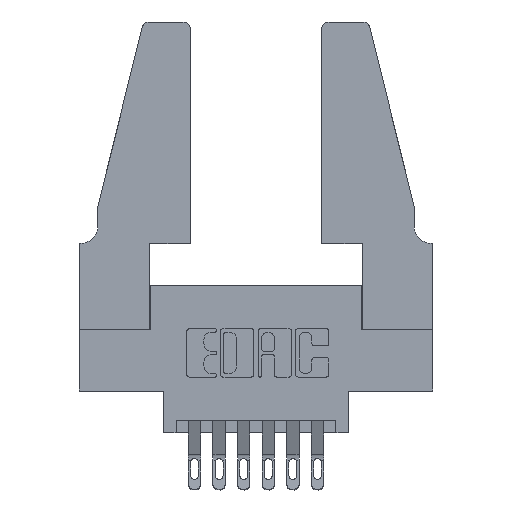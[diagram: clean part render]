
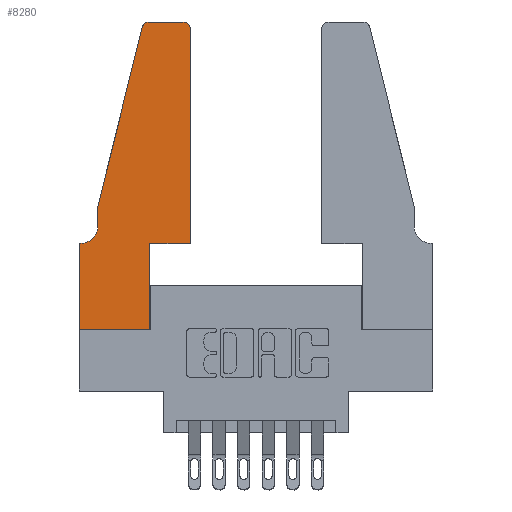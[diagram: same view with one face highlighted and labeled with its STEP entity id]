
A CAD part, top view. The second image highlights one B-rep face of the part: STEP entity #8280.
In plain terms, the highlighted planar face has unit normal (0, 0, 1).
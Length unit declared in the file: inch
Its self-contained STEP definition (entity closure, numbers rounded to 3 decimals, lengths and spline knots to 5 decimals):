
#28 = VECTOR ( 'NONE', #270, 39.37008 ) ;
#76 = CIRCLE ( 'NONE', #6480, 0.03 ) ;
#229 = VERTEX_POINT ( 'NONE', #832 ) ;
#270 = DIRECTION ( 'NONE',  ( -0.239, -0.971, 0. ) ) ;
#282 = CARTESIAN_POINT ( 'NONE',  ( 0.0755, 0.5, 0.37 ) ) ;
#546 = LINE ( 'NONE', #2234, #886 ) ;
#561 = CARTESIAN_POINT ( 'NONE',  ( 0.2865, 0.35, 0.37 ) ) ;
#663 = VERTEX_POINT ( 'NONE', #5382 ) ;
#832 = CARTESIAN_POINT ( 'NONE',  ( 0.0755, 0.5, 0.37 ) ) ;
#846 = EDGE_CURVE ( 'NONE', #4958, #2018, #1470, .T. ) ;
#886 = VECTOR ( 'NONE', #2014, 39.37008 ) ;
#1030 = CARTESIAN_POINT ( 'NONE',  ( 0., 0.35, 0.37 ) ) ;
#1070 = ORIENTED_EDGE ( 'NONE', *, *, #9901, .T. ) ;
#1349 = VERTEX_POINT ( 'NONE', #561 ) ;
#1470 = LINE ( 'NONE', #11175, #6587 ) ;
#1544 = CARTESIAN_POINT ( 'NONE',  ( 0., 0.35, 0.37 ) ) ;
#1828 = ORIENTED_EDGE ( 'NONE', *, *, #3457, .T. ) ;
#1980 = DIRECTION ( 'NONE',  ( 0., 0., 1. ) ) ;
#2014 = DIRECTION ( 'NONE',  ( 1., 0., 0. ) ) ;
#2018 = VERTEX_POINT ( 'NONE', #7137 ) ;
#2154 = CARTESIAN_POINT ( 'NONE',  ( 0.0755, 0.42, 0.37 ) ) ;
#2234 = CARTESIAN_POINT ( 'NONE',  ( 0.4505, 0.35, 0.37 ) ) ;
#2281 = CARTESIAN_POINT ( 'NONE',  ( 0.4205, 1.22, 0.37 ) ) ;
#2283 = EDGE_LOOP ( 'NONE', ( #7116, #5457, #11594, #6829, #2552, #1828, #3752, #1070, #11654, #7607, #7612, #5380 ) ) ;
#2552 = ORIENTED_EDGE ( 'NONE', *, *, #4935, .T. ) ;
#2632 = CIRCLE ( 'NONE', #11455, 0.03 ) ;
#2892 = DIRECTION ( 'NONE',  ( -1., 0., 0. ) ) ;
#2947 = VERTEX_POINT ( 'NONE', #3494 ) ;
#2970 = CARTESIAN_POINT ( 'NONE',  ( 0.0055, 0.42, 0.37 ) ) ;
#3032 = DIRECTION ( 'NONE',  ( 0., -1., 0. ) ) ;
#3078 = DIRECTION ( 'NONE',  ( 0., 0., -1. ) ) ;
#3112 = CARTESIAN_POINT ( 'NONE',  ( 0.25487, 1.22718, 0.37 ) ) ;
#3214 = DIRECTION ( 'NONE',  ( 1., 0., 0. ) ) ;
#3267 = EDGE_CURVE ( 'NONE', #663, #5713, #5959, .T. ) ;
#3369 = LINE ( 'NONE', #282, #28 ) ;
#3457 = EDGE_CURVE ( 'NONE', #9056, #4958, #6723, .T. ) ;
#3494 = CARTESIAN_POINT ( 'NONE',  ( 0.4505, 0.35, 0.37 ) ) ;
#3605 = AXIS2_PLACEMENT_3D ( 'NONE', #1030, #4929, #11365 ) ;
#3752 = ORIENTED_EDGE ( 'NONE', *, *, #846, .T. ) ;
#4354 = FACE_OUTER_BOUND ( 'NONE', #2283, .T. ) ;
#4867 = EDGE_CURVE ( 'NONE', #1349, #2947, #546, .T. ) ;
#4929 = DIRECTION ( 'NONE',  ( 0., 0., 1. ) ) ;
#4935 = EDGE_CURVE ( 'NONE', #7271, #9056, #5158, .T. ) ;
#4958 = VERTEX_POINT ( 'NONE', #1544 ) ;
#5158 = CIRCLE ( 'NONE', #7493, 0.07 ) ;
#5163 = EDGE_CURVE ( 'NONE', #5981, #229, #3369, .T. ) ;
#5170 = DIRECTION ( 'NONE',  ( 0., 1., 0. ) ) ;
#5186 = LINE ( 'NONE', #6149, #9880 ) ;
#5211 = VECTOR ( 'NONE', #7538, 39.37008 ) ;
#5380 = ORIENTED_EDGE ( 'NONE', *, *, #5427, .T. ) ;
#5382 = CARTESIAN_POINT ( 'NONE',  ( 0.4205, 1.25, 0.37 ) ) ;
#5427 = EDGE_CURVE ( 'NONE', #6000, #663, #2632, .T. ) ;
#5457 = ORIENTED_EDGE ( 'NONE', *, *, #10553, .T. ) ;
#5499 = VECTOR ( 'NONE', #5170, 39.37008 ) ;
#5713 = VERTEX_POINT ( 'NONE', #11856 ) ;
#5959 = LINE ( 'NONE', #8402, #10574 ) ;
#5981 = VERTEX_POINT ( 'NONE', #3112 ) ;
#6000 = VERTEX_POINT ( 'NONE', #6984 ) ;
#6149 = CARTESIAN_POINT ( 'NONE',  ( 0.0755, 0.5, 0.37 ) ) ;
#6259 = CARTESIAN_POINT ( 'NONE',  ( 0.4505, 0.35, 0.37 ) ) ;
#6480 = AXIS2_PLACEMENT_3D ( 'NONE', #7685, #1980, #8608 ) ;
#6587 = VECTOR ( 'NONE', #3032, 39.37008 ) ;
#6723 = LINE ( 'NONE', #10521, #8886 ) ;
#6829 = ORIENTED_EDGE ( 'NONE', *, *, #10794, .T. ) ;
#6984 = CARTESIAN_POINT ( 'NONE',  ( 0.4505, 1.22, 0.37 ) ) ;
#7116 = ORIENTED_EDGE ( 'NONE', *, *, #3267, .T. ) ;
#7130 = DIRECTION ( 'NONE',  ( 0., -1., 0. ) ) ;
#7137 = CARTESIAN_POINT ( 'NONE',  ( 0., 0., 0.37 ) ) ;
#7271 = VERTEX_POINT ( 'NONE', #2154 ) ;
#7493 = AXIS2_PLACEMENT_3D ( 'NONE', #2970, #3078, #2892 ) ;
#7524 = VERTEX_POINT ( 'NONE', #11751 ) ;
#7538 = DIRECTION ( 'NONE',  ( 1., 0., 0. ) ) ;
#7607 = ORIENTED_EDGE ( 'NONE', *, *, #4867, .T. ) ;
#7612 = ORIENTED_EDGE ( 'NONE', *, *, #8497, .T. ) ;
#7685 = CARTESIAN_POINT ( 'NONE',  ( 0.284, 1.22, 0.37 ) ) ;
#8007 = CARTESIAN_POINT ( 'NONE',  ( 0.2865, 0.35, 0.37 ) ) ;
#8021 = LINE ( 'NONE', #8007, #5499 ) ;
#8045 = LINE ( 'NONE', #9336, #5211 ) ;
#8280 = ADVANCED_FACE ( 'NONE', ( #4354 ), #10504, .T. ) ;
#8402 = CARTESIAN_POINT ( 'NONE',  ( 0.2605, 1.25, 0.37 ) ) ;
#8497 = EDGE_CURVE ( 'NONE', #2947, #6000, #11272, .T. ) ;
#8608 = DIRECTION ( 'NONE',  ( 1., 0., 0. ) ) ;
#8883 = DIRECTION ( 'NONE',  ( 0., 0., 1. ) ) ;
#8886 = VECTOR ( 'NONE', #10641, 39.37008 ) ;
#8923 = VECTOR ( 'NONE', #10816, 39.37008 ) ;
#9056 = VERTEX_POINT ( 'NONE', #9799 ) ;
#9336 = CARTESIAN_POINT ( 'NONE',  ( 0., 0., 0.37 ) ) ;
#9799 = CARTESIAN_POINT ( 'NONE',  ( 0.0055, 0.35, 0.37 ) ) ;
#9880 = VECTOR ( 'NONE', #7130, 39.37008 ) ;
#9901 = EDGE_CURVE ( 'NONE', #2018, #7524, #8045, .T. ) ;
#10504 = PLANE ( 'NONE',  #3605 ) ;
#10521 = CARTESIAN_POINT ( 'NONE',  ( 0.0755, 0.35, 0.37 ) ) ;
#10553 = EDGE_CURVE ( 'NONE', #5713, #5981, #76, .T. ) ;
#10574 = VECTOR ( 'NONE', #11727, 39.37008 ) ;
#10641 = DIRECTION ( 'NONE',  ( -1., 0., 0. ) ) ;
#10779 = EDGE_CURVE ( 'NONE', #7524, #1349, #8021, .T. ) ;
#10794 = EDGE_CURVE ( 'NONE', #229, #7271, #5186, .T. ) ;
#10816 = DIRECTION ( 'NONE',  ( 0., 1., 0. ) ) ;
#11175 = CARTESIAN_POINT ( 'NONE',  ( 0., 0., 0.37 ) ) ;
#11272 = LINE ( 'NONE', #6259, #8923 ) ;
#11365 = DIRECTION ( 'NONE',  ( 1., 0., 0. ) ) ;
#11455 = AXIS2_PLACEMENT_3D ( 'NONE', #2281, #8883, #3214 ) ;
#11594 = ORIENTED_EDGE ( 'NONE', *, *, #5163, .T. ) ;
#11654 = ORIENTED_EDGE ( 'NONE', *, *, #10779, .T. ) ;
#11727 = DIRECTION ( 'NONE',  ( -1., 0., 0. ) ) ;
#11751 = CARTESIAN_POINT ( 'NONE',  ( 0.2865, 0., 0.37 ) ) ;
#11856 = CARTESIAN_POINT ( 'NONE',  ( 0.284, 1.25, 0.37 ) ) ;
